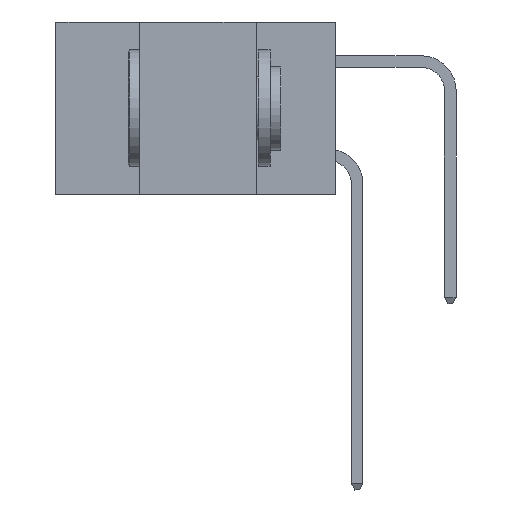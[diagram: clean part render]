
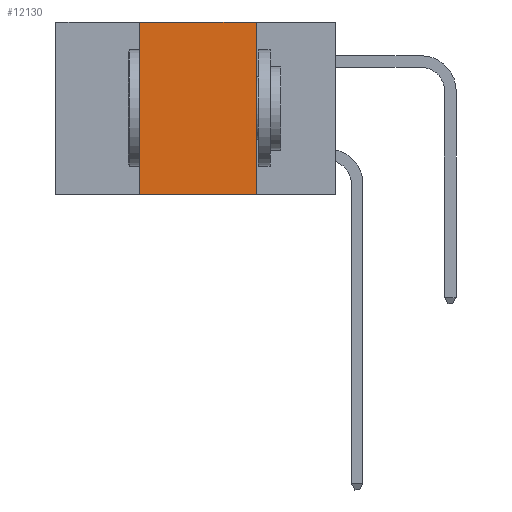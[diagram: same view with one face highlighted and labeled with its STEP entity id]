
A CAD part, left-side view. The second image highlights one B-rep face of the part: STEP entity #12130.
In plain terms, the highlighted planar face has unit normal (-1, 0, 0).
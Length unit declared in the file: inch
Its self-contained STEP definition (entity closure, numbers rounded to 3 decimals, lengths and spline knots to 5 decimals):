
#36 = CARTESIAN_POINT ( 'NONE',  ( 0., 0.6, -0.37 ) ) ;
#1090 = AXIS2_PLACEMENT_3D ( 'NONE', #18179, #8137, #13038 ) ;
#1262 = ORIENTED_EDGE ( 'NONE', *, *, #14064, .F. ) ;
#1341 = LINE ( 'NONE', #4334, #14182 ) ;
#1385 = VECTOR ( 'NONE', #6215, 39.37008 ) ;
#1694 = CARTESIAN_POINT ( 'NONE',  ( 0., 0.6, 0. ) ) ;
#3528 = DIRECTION ( 'NONE',  ( 0., -1., 0. ) ) ;
#4334 = CARTESIAN_POINT ( 'NONE',  ( 0., 0.17, 0. ) ) ;
#4536 = EDGE_CURVE ( 'NONE', #6262, #6567, #10224, .T. ) ;
#5211 = VECTOR ( 'NONE', #6988, 39.37008 ) ;
#5398 = EDGE_LOOP ( 'NONE', ( #17668, #1262, #16836, #7527 ) ) ;
#6215 = DIRECTION ( 'NONE',  ( 0., 0., 1. ) ) ;
#6262 = VERTEX_POINT ( 'NONE', #11984 ) ;
#6567 = VERTEX_POINT ( 'NONE', #10799 ) ;
#6642 = FACE_OUTER_BOUND ( 'NONE', #5398, .T. ) ;
#6988 = DIRECTION ( 'NONE',  ( 0., -1., 0. ) ) ;
#7527 = ORIENTED_EDGE ( 'NONE', *, *, #4536, .T. ) ;
#7607 = EDGE_CURVE ( 'NONE', #16053, #6567, #1341, .T. ) ;
#8137 = DIRECTION ( 'NONE',  ( 1., 0., 0. ) ) ;
#8943 = VECTOR ( 'NONE', #3528, 39.37008 ) ;
#9327 = CARTESIAN_POINT ( 'NONE',  ( 0., 0.42, 0. ) ) ;
#10224 = LINE ( 'NONE', #36, #5211 ) ;
#10334 = LINE ( 'NONE', #12642, #1385 ) ;
#10799 = CARTESIAN_POINT ( 'NONE',  ( 0., 0.17, -0.37 ) ) ;
#11279 = CARTESIAN_POINT ( 'NONE',  ( 0., 0.17, 0. ) ) ;
#11984 = CARTESIAN_POINT ( 'NONE',  ( 0., 0.42, -0.37 ) ) ;
#12130 = ADVANCED_FACE ( 'NONE', ( #6642 ), #16340, .F. ) ;
#12642 = CARTESIAN_POINT ( 'NONE',  ( 0., 0.42, 0. ) ) ;
#13038 = DIRECTION ( 'NONE',  ( 0., 0., -1. ) ) ;
#13083 = VERTEX_POINT ( 'NONE', #9327 ) ;
#13212 = EDGE_CURVE ( 'NONE', #6262, #13083, #10334, .T. ) ;
#13412 = LINE ( 'NONE', #1694, #8943 ) ;
#14064 = EDGE_CURVE ( 'NONE', #13083, #16053, #13412, .T. ) ;
#14182 = VECTOR ( 'NONE', #17698, 39.37008 ) ;
#16053 = VERTEX_POINT ( 'NONE', #11279 ) ;
#16340 = PLANE ( 'NONE',  #1090 ) ;
#16836 = ORIENTED_EDGE ( 'NONE', *, *, #13212, .F. ) ;
#17668 = ORIENTED_EDGE ( 'NONE', *, *, #7607, .F. ) ;
#17698 = DIRECTION ( 'NONE',  ( 0., 0., -1. ) ) ;
#18179 = CARTESIAN_POINT ( 'NONE',  ( 0., 0.6, 0. ) ) ;
